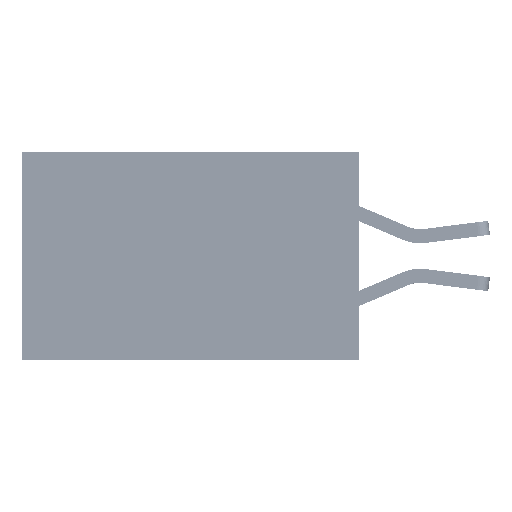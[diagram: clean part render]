
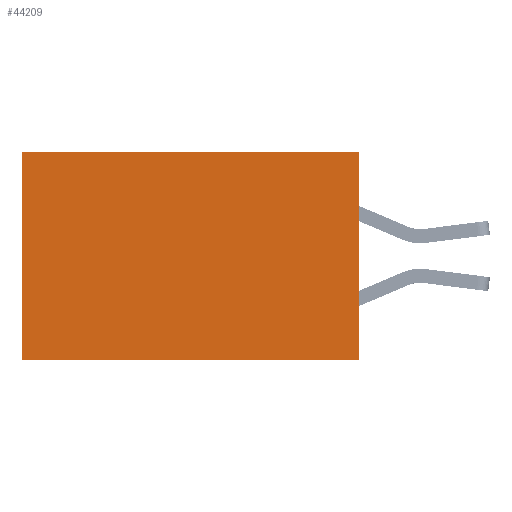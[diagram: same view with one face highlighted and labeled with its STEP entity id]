
A CAD part, left-side view. The second image highlights one B-rep face of the part: STEP entity #44209.
In plain terms, the highlighted planar face has unit normal (-1, 0, 0).
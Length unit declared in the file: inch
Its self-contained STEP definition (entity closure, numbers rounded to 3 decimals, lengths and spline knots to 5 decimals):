
#405 = CARTESIAN_POINT ( 'NONE',  ( 0.2875, 0.6, 0. ) ) ;
#1324 = VECTOR ( 'NONE', #6287, 39.37008 ) ;
#2551 = CARTESIAN_POINT ( 'NONE',  ( 0.2875, 0., 0. ) ) ;
#4603 = ORIENTED_EDGE ( 'NONE', *, *, #11363, .T. ) ;
#6287 = DIRECTION ( 'NONE',  ( 0., 1., 0. ) ) ;
#6731 = EDGE_LOOP ( 'NONE', ( #12067, #48089, #32785, #4603 ) ) ;
#8343 = EDGE_CURVE ( 'NONE', #37999, #40805, #31747, .T. ) ;
#11363 = EDGE_CURVE ( 'NONE', #40744, #14590, #14000, .T. ) ;
#11921 = DIRECTION ( 'NONE',  ( 0., 0., -1. ) ) ;
#12067 = ORIENTED_EDGE ( 'NONE', *, *, #33080, .T. ) ;
#13631 = LINE ( 'NONE', #16867, #16059 ) ;
#14000 = LINE ( 'NONE', #2551, #1324 ) ;
#14590 = VERTEX_POINT ( 'NONE', #37692 ) ;
#16059 = VECTOR ( 'NONE', #44313, 39.37008 ) ;
#16867 = CARTESIAN_POINT ( 'NONE',  ( 0.2875, 0., 0. ) ) ;
#19188 = CARTESIAN_POINT ( 'NONE',  ( 0.2875, 0., -0.37 ) ) ;
#20232 = CARTESIAN_POINT ( 'NONE',  ( 0.2875, 0., 0. ) ) ;
#21258 = CARTESIAN_POINT ( 'NONE',  ( 0.2875, 0., 0. ) ) ;
#22976 = FACE_OUTER_BOUND ( 'NONE', #6731, .T. ) ;
#25145 = DIRECTION ( 'NONE',  ( 0., 0., -1. ) ) ;
#25765 = VECTOR ( 'NONE', #46113, 39.37008 ) ;
#27074 = LINE ( 'NONE', #405, #48787 ) ;
#31747 = LINE ( 'NONE', #19188, #25765 ) ;
#32785 = ORIENTED_EDGE ( 'NONE', *, *, #32857, .F. ) ;
#32857 = EDGE_CURVE ( 'NONE', #40744, #37999, #13631, .T. ) ;
#33080 = EDGE_CURVE ( 'NONE', #14590, #40805, #27074, .T. ) ;
#35547 = CARTESIAN_POINT ( 'NONE',  ( 0.2875, 0.6, -0.37 ) ) ;
#37692 = CARTESIAN_POINT ( 'NONE',  ( 0.2875, 0.6, 0. ) ) ;
#37999 = VERTEX_POINT ( 'NONE', #42265 ) ;
#39016 = AXIS2_PLACEMENT_3D ( 'NONE', #21258, #48209, #25145 ) ;
#40744 = VERTEX_POINT ( 'NONE', #20232 ) ;
#40805 = VERTEX_POINT ( 'NONE', #35547 ) ;
#41304 = PLANE ( 'NONE',  #39016 ) ;
#42265 = CARTESIAN_POINT ( 'NONE',  ( 0.2875, 0., -0.37 ) ) ;
#44209 = ADVANCED_FACE ( 'NONE', ( #22976 ), #41304, .F. ) ;
#44313 = DIRECTION ( 'NONE',  ( 0., 0., -1. ) ) ;
#46113 = DIRECTION ( 'NONE',  ( 0., 1., 0. ) ) ;
#48089 = ORIENTED_EDGE ( 'NONE', *, *, #8343, .F. ) ;
#48209 = DIRECTION ( 'NONE',  ( 1., 0., 0. ) ) ;
#48787 = VECTOR ( 'NONE', #11921, 39.37008 ) ;
